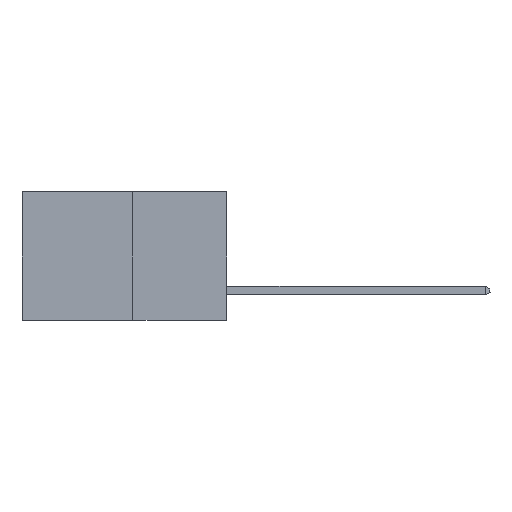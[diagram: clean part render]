
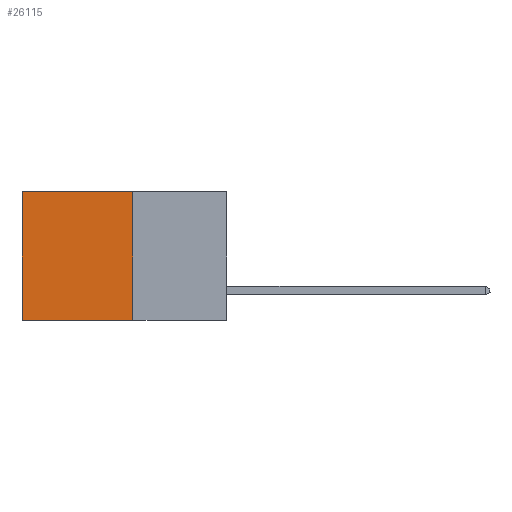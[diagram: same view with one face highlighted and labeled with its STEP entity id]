
A CAD part, left-side view. The second image highlights one B-rep face of the part: STEP entity #26115.
In plain terms, the highlighted planar face has unit normal (-1, 0, 0).
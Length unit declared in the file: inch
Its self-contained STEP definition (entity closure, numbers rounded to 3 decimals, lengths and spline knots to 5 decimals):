
#636 = EDGE_CURVE ( 'NONE', #20778, #23820, #4979, .T. ) ;
#679 = EDGE_CURVE ( 'NONE', #16905, #13638, #19963, .T. ) ;
#1779 = CARTESIAN_POINT ( 'NONE',  ( 0.277, 0.59, -0.37 ) ) ;
#2502 = PLANE ( 'NONE',  #4428 ) ;
#3640 = VECTOR ( 'NONE', #23081, 39.37008 ) ;
#4428 = AXIS2_PLACEMENT_3D ( 'NONE', #20951, #8772, #22946 ) ;
#4639 = CARTESIAN_POINT ( 'NONE',  ( 0.277, 0.27, 0. ) ) ;
#4979 = LINE ( 'NONE', #13562, #15856 ) ;
#6705 = EDGE_CURVE ( 'NONE', #20778, #16905, #7495, .T. ) ;
#6865 = VECTOR ( 'NONE', #16209, 39.37008 ) ;
#7260 = EDGE_LOOP ( 'NONE', ( #13240, #23995, #18346, #20257 ) ) ;
#7495 = LINE ( 'NONE', #16384, #6865 ) ;
#7669 = LINE ( 'NONE', #19045, #12497 ) ;
#8772 = DIRECTION ( 'NONE',  ( 1., 0., 0. ) ) ;
#9057 = EDGE_CURVE ( 'NONE', #23820, #13638, #7669, .T. ) ;
#10915 = FACE_OUTER_BOUND ( 'NONE', #7260, .T. ) ;
#11399 = DIRECTION ( 'NONE',  ( 0., 1., 0. ) ) ;
#12497 = VECTOR ( 'NONE', #18516, 39.37008 ) ;
#13240 = ORIENTED_EDGE ( 'NONE', *, *, #9057, .T. ) ;
#13562 = CARTESIAN_POINT ( 'NONE',  ( 0.277, 0.27, 0. ) ) ;
#13638 = VERTEX_POINT ( 'NONE', #1779 ) ;
#14723 = CARTESIAN_POINT ( 'NONE',  ( 0.277, 0.27, -0.37 ) ) ;
#15856 = VECTOR ( 'NONE', #11399, 39.37008 ) ;
#16209 = DIRECTION ( 'NONE',  ( 0., 0., -1. ) ) ;
#16384 = CARTESIAN_POINT ( 'NONE',  ( 0.277, 0.27, -0.37 ) ) ;
#16905 = VERTEX_POINT ( 'NONE', #14723 ) ;
#18346 = ORIENTED_EDGE ( 'NONE', *, *, #6705, .F. ) ;
#18516 = DIRECTION ( 'NONE',  ( 0., 0., -1. ) ) ;
#19045 = CARTESIAN_POINT ( 'NONE',  ( 0.277, 0.59, -0.37 ) ) ;
#19963 = LINE ( 'NONE', #21769, #3640 ) ;
#20257 = ORIENTED_EDGE ( 'NONE', *, *, #636, .T. ) ;
#20778 = VERTEX_POINT ( 'NONE', #4639 ) ;
#20951 = CARTESIAN_POINT ( 'NONE',  ( 0.277, 0.27, -0.37 ) ) ;
#21220 = CARTESIAN_POINT ( 'NONE',  ( 0.277, 0.59, 0. ) ) ;
#21769 = CARTESIAN_POINT ( 'NONE',  ( 0.277, 0.27, -0.37 ) ) ;
#22946 = DIRECTION ( 'NONE',  ( 0., 0., -1. ) ) ;
#23081 = DIRECTION ( 'NONE',  ( 0., 1., 0. ) ) ;
#23820 = VERTEX_POINT ( 'NONE', #21220 ) ;
#23995 = ORIENTED_EDGE ( 'NONE', *, *, #679, .F. ) ;
#26115 = ADVANCED_FACE ( 'NONE', ( #10915 ), #2502, .F. ) ;
